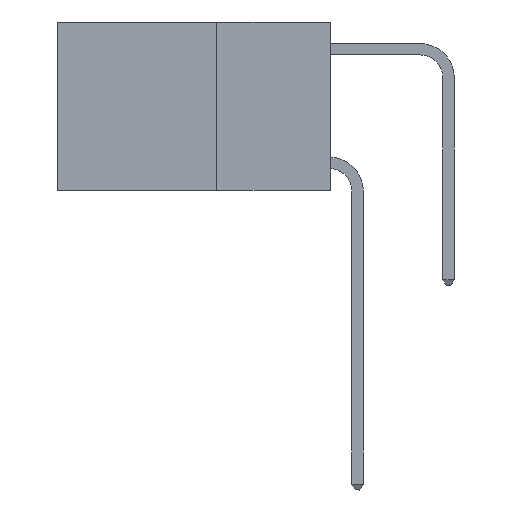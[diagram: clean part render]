
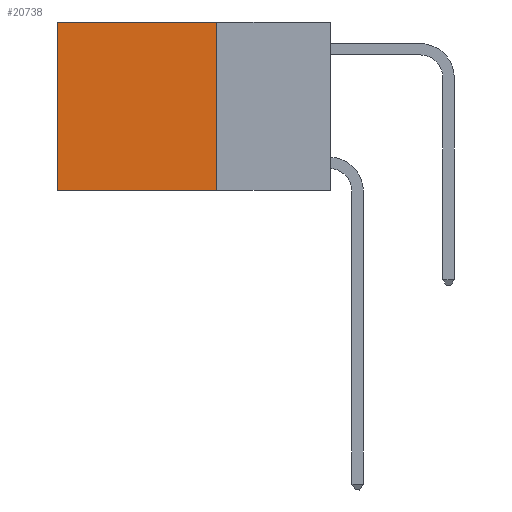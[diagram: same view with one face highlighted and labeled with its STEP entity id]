
A CAD part, left-side view. The second image highlights one B-rep face of the part: STEP entity #20738.
In plain terms, the highlighted planar face has unit normal (-1, 0, 0).
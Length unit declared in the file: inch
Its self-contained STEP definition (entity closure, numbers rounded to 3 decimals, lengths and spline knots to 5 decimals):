
#370 = VERTEX_POINT ( 'NONE', #11233 ) ;
#650 = VECTOR ( 'NONE', #4191, 39.37008 ) ;
#2922 = CARTESIAN_POINT ( 'NONE',  ( 0.2625, 0.6, 0. ) ) ;
#4180 = EDGE_CURVE ( 'NONE', #7054, #4730, #23093, .T. ) ;
#4191 = DIRECTION ( 'NONE',  ( 0., 0., -1. ) ) ;
#4368 = LINE ( 'NONE', #17746, #6732 ) ;
#4497 = VECTOR ( 'NONE', #15313, 39.37008 ) ;
#4730 = VERTEX_POINT ( 'NONE', #10687 ) ;
#6732 = VECTOR ( 'NONE', #12349, 39.37008 ) ;
#6986 = LINE ( 'NONE', #21625, #7699 ) ;
#7006 = DIRECTION ( 'NONE',  ( 0., 0., -1. ) ) ;
#7054 = VERTEX_POINT ( 'NONE', #7293 ) ;
#7293 = CARTESIAN_POINT ( 'NONE',  ( 0.2625, 0.25, -0.37 ) ) ;
#7699 = VECTOR ( 'NONE', #12709, 39.37008 ) ;
#8745 = ORIENTED_EDGE ( 'NONE', *, *, #21125, .F. ) ;
#10687 = CARTESIAN_POINT ( 'NONE',  ( 0.2625, 0.6, -0.37 ) ) ;
#10989 = CARTESIAN_POINT ( 'NONE',  ( 0.2625, 0.25, 0. ) ) ;
#11059 = CARTESIAN_POINT ( 'NONE',  ( 0.2625, 0.6, 0. ) ) ;
#11209 = EDGE_CURVE ( 'NONE', #20306, #4730, #13508, .T. ) ;
#11233 = CARTESIAN_POINT ( 'NONE',  ( 0.2625, 0.25, 0. ) ) ;
#12267 = AXIS2_PLACEMENT_3D ( 'NONE', #10989, #22452, #7006 ) ;
#12313 = ORIENTED_EDGE ( 'NONE', *, *, #13556, .T. ) ;
#12349 = DIRECTION ( 'NONE',  ( 0., 0., -1. ) ) ;
#12709 = DIRECTION ( 'NONE',  ( 0., 1., 0. ) ) ;
#13508 = LINE ( 'NONE', #2922, #650 ) ;
#13556 = EDGE_CURVE ( 'NONE', #370, #20306, #6986, .T. ) ;
#14717 = ORIENTED_EDGE ( 'NONE', *, *, #11209, .T. ) ;
#15313 = DIRECTION ( 'NONE',  ( 0., 1., 0. ) ) ;
#16384 = FACE_OUTER_BOUND ( 'NONE', #16813, .T. ) ;
#16813 = EDGE_LOOP ( 'NONE', ( #14717, #17455, #8745, #12313 ) ) ;
#17455 = ORIENTED_EDGE ( 'NONE', *, *, #4180, .F. ) ;
#17746 = CARTESIAN_POINT ( 'NONE',  ( 0.2625, 0.25, 0. ) ) ;
#19403 = CARTESIAN_POINT ( 'NONE',  ( 0.2625, 0.25, -0.37 ) ) ;
#20306 = VERTEX_POINT ( 'NONE', #11059 ) ;
#20738 = ADVANCED_FACE ( 'NONE', ( #16384 ), #23953, .F. ) ;
#21125 = EDGE_CURVE ( 'NONE', #370, #7054, #4368, .T. ) ;
#21625 = CARTESIAN_POINT ( 'NONE',  ( 0.2625, 0.25, 0. ) ) ;
#22452 = DIRECTION ( 'NONE',  ( 1., 0., 0. ) ) ;
#23093 = LINE ( 'NONE', #19403, #4497 ) ;
#23953 = PLANE ( 'NONE',  #12267 ) ;
